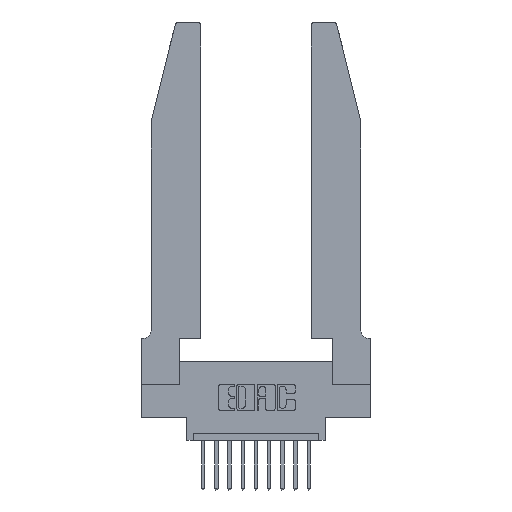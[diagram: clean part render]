
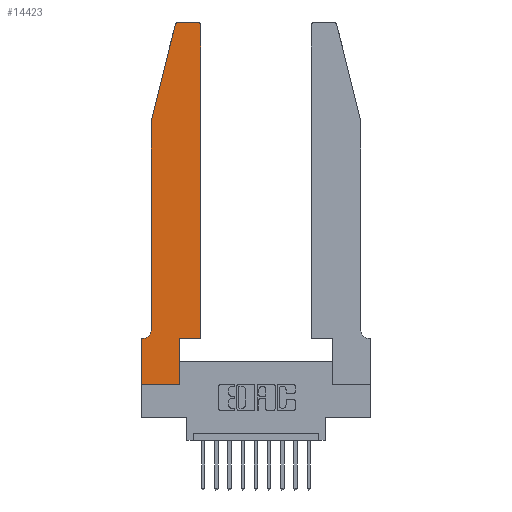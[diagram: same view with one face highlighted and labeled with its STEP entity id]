
A CAD part, top view. The second image highlights one B-rep face of the part: STEP entity #14423.
In plain terms, the highlighted planar face has unit normal (0, 0, 1).
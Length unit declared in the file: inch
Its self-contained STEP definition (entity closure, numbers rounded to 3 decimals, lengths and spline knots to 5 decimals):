
#92 = VERTEX_POINT ( 'NONE', #1109 ) ;
#179 = DIRECTION ( 'NONE',  ( 0., 0., 1. ) ) ;
#267 = VERTEX_POINT ( 'NONE', #287 ) ;
#287 = CARTESIAN_POINT ( 'NONE',  ( 0., 0., 0.37 ) ) ;
#314 = VERTEX_POINT ( 'NONE', #15459 ) ;
#451 = EDGE_CURVE ( 'NONE', #267, #14644, #10006, .T. ) ;
#536 = VECTOR ( 'NONE', #8367, 39.37008 ) ;
#615 = CARTESIAN_POINT ( 'NONE',  ( 0., 0.35, 0.37 ) ) ;
#725 = AXIS2_PLACEMENT_3D ( 'NONE', #13193, #3295, #4405 ) ;
#773 = DIRECTION ( 'NONE',  ( 0., 1., 0. ) ) ;
#1003 = DIRECTION ( 'NONE',  ( 0., 0., 1. ) ) ;
#1109 = CARTESIAN_POINT ( 'NONE',  ( 0.4205, 2.75, 0.37 ) ) ;
#1119 = DIRECTION ( 'NONE',  ( 1., 0., 0. ) ) ;
#1185 = LINE ( 'NONE', #2811, #11749 ) ;
#1408 = VERTEX_POINT ( 'NONE', #11349 ) ;
#1612 = FACE_OUTER_BOUND ( 'NONE', #5558, .T. ) ;
#1713 = EDGE_CURVE ( 'NONE', #92, #5142, #1185, .T. ) ;
#2154 = ORIENTED_EDGE ( 'NONE', *, *, #451, .T. ) ;
#2566 = VECTOR ( 'NONE', #7807, 39.37008 ) ;
#2811 = CARTESIAN_POINT ( 'NONE',  ( 0.2605, 2.75, 0.37 ) ) ;
#3008 = AXIS2_PLACEMENT_3D ( 'NONE', #3582, #1003, #1119 ) ;
#3063 = LINE ( 'NONE', #10619, #15505 ) ;
#3170 = DIRECTION ( 'NONE',  ( 0., -1., 0. ) ) ;
#3295 = DIRECTION ( 'NONE',  ( 0., 0., 1. ) ) ;
#3540 = VERTEX_POINT ( 'NONE', #15797 ) ;
#3582 = CARTESIAN_POINT ( 'NONE',  ( 0.4205, 2.72, 0.37 ) ) ;
#3796 = DIRECTION ( 'NONE',  ( 0., 1., 0. ) ) ;
#3803 = EDGE_CURVE ( 'NONE', #14644, #3540, #10255, .T. ) ;
#3808 = CARTESIAN_POINT ( 'NONE',  ( 0.4505, 0.35, 0.37 ) ) ;
#3871 = DIRECTION ( 'NONE',  ( 0., 0., -1. ) ) ;
#4051 = VERTEX_POINT ( 'NONE', #4874 ) ;
#4199 = ORIENTED_EDGE ( 'NONE', *, *, #3803, .T. ) ;
#4405 = DIRECTION ( 'NONE',  ( 1., 0., 0. ) ) ;
#4430 = ORIENTED_EDGE ( 'NONE', *, *, #8452, .T. ) ;
#4531 = EDGE_CURVE ( 'NONE', #8251, #10684, #8833, .T. ) ;
#4557 = VECTOR ( 'NONE', #3170, 39.37008 ) ;
#4871 = LINE ( 'NONE', #14845, #10523 ) ;
#4874 = CARTESIAN_POINT ( 'NONE',  ( 0.0055, 0.35, 0.37 ) ) ;
#5130 = CIRCLE ( 'NONE', #12943, 0.07 ) ;
#5142 = VERTEX_POINT ( 'NONE', #9912 ) ;
#5262 = DIRECTION ( 'NONE',  ( -1., 0., 0. ) ) ;
#5468 = CARTESIAN_POINT ( 'NONE',  ( 0., 0., 0.37 ) ) ;
#5558 = EDGE_LOOP ( 'NONE', ( #15402, #7625, #4430, #6352, #6499, #9654, #10669, #2154, #4199, #15174, #8834, #12220 ) ) ;
#5869 = CARTESIAN_POINT ( 'NONE',  ( 0.0755, 2., 0.37 ) ) ;
#5903 = EDGE_CURVE ( 'NONE', #15864, #267, #7836, .T. ) ;
#5945 = VECTOR ( 'NONE', #773, 39.37008 ) ;
#6010 = CARTESIAN_POINT ( 'NONE',  ( 0., 0., 0.37 ) ) ;
#6346 = CARTESIAN_POINT ( 'NONE',  ( 0.4505, 0.35, 0.37 ) ) ;
#6352 = ORIENTED_EDGE ( 'NONE', *, *, #9389, .T. ) ;
#6499 = ORIENTED_EDGE ( 'NONE', *, *, #6529, .T. ) ;
#6529 = EDGE_CURVE ( 'NONE', #6829, #4051, #5130, .T. ) ;
#6829 = VERTEX_POINT ( 'NONE', #10569 ) ;
#7160 = LINE ( 'NONE', #5869, #536 ) ;
#7400 = EDGE_CURVE ( 'NONE', #3540, #8251, #8771, .T. ) ;
#7469 = VECTOR ( 'NONE', #3796, 39.37008 ) ;
#7625 = ORIENTED_EDGE ( 'NONE', *, *, #15793, .T. ) ;
#7807 = DIRECTION ( 'NONE',  ( 1., 0., 0. ) ) ;
#7836 = LINE ( 'NONE', #5468, #4557 ) ;
#8251 = VERTEX_POINT ( 'NONE', #3808 ) ;
#8354 = CIRCLE ( 'NONE', #725, 0.03 ) ;
#8367 = DIRECTION ( 'NONE',  ( 0., -1., 0. ) ) ;
#8452 = EDGE_CURVE ( 'NONE', #1408, #314, #4871, .T. ) ;
#8771 = LINE ( 'NONE', #11569, #2566 ) ;
#8833 = LINE ( 'NONE', #6346, #7469 ) ;
#8834 = ORIENTED_EDGE ( 'NONE', *, *, #4531, .T. ) ;
#9389 = EDGE_CURVE ( 'NONE', #314, #6829, #7160, .T. ) ;
#9654 = ORIENTED_EDGE ( 'NONE', *, *, #9897, .T. ) ;
#9844 = DIRECTION ( 'NONE',  ( -0.239, -0.971, 0. ) ) ;
#9897 = EDGE_CURVE ( 'NONE', #4051, #15864, #3063, .T. ) ;
#9912 = CARTESIAN_POINT ( 'NONE',  ( 0.284, 2.75, 0.37 ) ) ;
#10006 = LINE ( 'NONE', #6010, #14108 ) ;
#10064 = CARTESIAN_POINT ( 'NONE',  ( 0.0055, 0.42, 0.37 ) ) ;
#10255 = LINE ( 'NONE', #15846, #5945 ) ;
#10523 = VECTOR ( 'NONE', #9844, 39.37008 ) ;
#10569 = CARTESIAN_POINT ( 'NONE',  ( 0.0755, 0.42, 0.37 ) ) ;
#10619 = CARTESIAN_POINT ( 'NONE',  ( 0.0755, 0.35, 0.37 ) ) ;
#10669 = ORIENTED_EDGE ( 'NONE', *, *, #5903, .T. ) ;
#10684 = VERTEX_POINT ( 'NONE', #12003 ) ;
#11349 = CARTESIAN_POINT ( 'NONE',  ( 0.25487, 2.72718, 0.37 ) ) ;
#11443 = DIRECTION ( 'NONE',  ( 1., 0., 0. ) ) ;
#11569 = CARTESIAN_POINT ( 'NONE',  ( 0.4505, 0.35, 0.37 ) ) ;
#11749 = VECTOR ( 'NONE', #5262, 39.37008 ) ;
#12003 = CARTESIAN_POINT ( 'NONE',  ( 0.4505, 2.72, 0.37 ) ) ;
#12220 = ORIENTED_EDGE ( 'NONE', *, *, #12976, .T. ) ;
#12737 = DIRECTION ( 'NONE',  ( -1., 0., 0. ) ) ;
#12919 = CARTESIAN_POINT ( 'NONE',  ( 0.2865, 0., 0.37 ) ) ;
#12943 = AXIS2_PLACEMENT_3D ( 'NONE', #10064, #3871, #12737 ) ;
#12976 = EDGE_CURVE ( 'NONE', #10684, #92, #15441, .T. ) ;
#13033 = AXIS2_PLACEMENT_3D ( 'NONE', #15302, #179, #11443 ) ;
#13193 = CARTESIAN_POINT ( 'NONE',  ( 0.284, 2.72, 0.37 ) ) ;
#14030 = PLANE ( 'NONE',  #13033 ) ;
#14108 = VECTOR ( 'NONE', #14729, 39.37008 ) ;
#14155 = DIRECTION ( 'NONE',  ( -1., 0., 0. ) ) ;
#14423 = ADVANCED_FACE ( 'NONE', ( #1612 ), #14030, .T. ) ;
#14644 = VERTEX_POINT ( 'NONE', #12919 ) ;
#14729 = DIRECTION ( 'NONE',  ( 1., 0., 0. ) ) ;
#14845 = CARTESIAN_POINT ( 'NONE',  ( 0.0755, 2., 0.37 ) ) ;
#15174 = ORIENTED_EDGE ( 'NONE', *, *, #7400, .T. ) ;
#15302 = CARTESIAN_POINT ( 'NONE',  ( 0., 0.35, 0.37 ) ) ;
#15402 = ORIENTED_EDGE ( 'NONE', *, *, #1713, .T. ) ;
#15441 = CIRCLE ( 'NONE', #3008, 0.03 ) ;
#15459 = CARTESIAN_POINT ( 'NONE',  ( 0.0755, 2., 0.37 ) ) ;
#15505 = VECTOR ( 'NONE', #14155, 39.37008 ) ;
#15793 = EDGE_CURVE ( 'NONE', #5142, #1408, #8354, .T. ) ;
#15797 = CARTESIAN_POINT ( 'NONE',  ( 0.2865, 0.35, 0.37 ) ) ;
#15846 = CARTESIAN_POINT ( 'NONE',  ( 0.2865, 0.35, 0.37 ) ) ;
#15864 = VERTEX_POINT ( 'NONE', #615 ) ;
